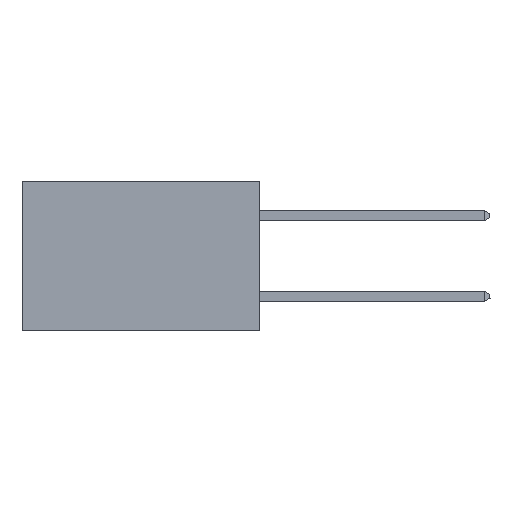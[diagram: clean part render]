
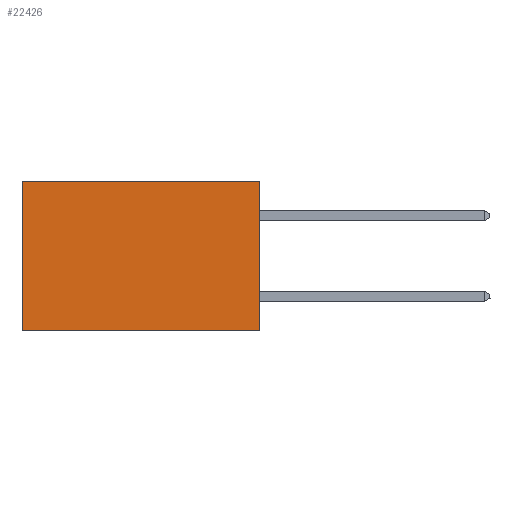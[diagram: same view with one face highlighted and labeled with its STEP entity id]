
A CAD part, left-side view. The second image highlights one B-rep face of the part: STEP entity #22426.
In plain terms, the highlighted planar face has unit normal (-1, 0, 0).
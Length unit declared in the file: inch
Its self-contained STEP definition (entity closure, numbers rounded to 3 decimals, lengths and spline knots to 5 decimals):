
#252 = DIRECTION ( 'NONE',  ( 0., 0., -1. ) ) ;
#736 = VECTOR ( 'NONE', #252, 39.37008 ) ;
#1738 = CARTESIAN_POINT ( 'NONE',  ( 0.277, 0., -0.37 ) ) ;
#1984 = CARTESIAN_POINT ( 'NONE',  ( 0.277, 0., 0. ) ) ;
#2696 = CARTESIAN_POINT ( 'NONE',  ( 0.277, 0.59, -0.37 ) ) ;
#3974 = PLANE ( 'NONE',  #16552 ) ;
#6568 = DIRECTION ( 'NONE',  ( 1., 0., 0. ) ) ;
#7200 = VECTOR ( 'NONE', #10506, 39.37008 ) ;
#7933 = CARTESIAN_POINT ( 'NONE',  ( 0.277, 0., -0.37 ) ) ;
#8193 = CARTESIAN_POINT ( 'NONE',  ( 0.277, 0.59, 0. ) ) ;
#9476 = DIRECTION ( 'NONE',  ( 0., 1., 0. ) ) ;
#10140 = VERTEX_POINT ( 'NONE', #2696 ) ;
#10506 = DIRECTION ( 'NONE',  ( 0., 0., -1. ) ) ;
#10649 = VERTEX_POINT ( 'NONE', #8193 ) ;
#10927 = EDGE_CURVE ( 'NONE', #25287, #30603, #21555, .T. ) ;
#11053 = ORIENTED_EDGE ( 'NONE', *, *, #25006, .T. ) ;
#11195 = EDGE_LOOP ( 'NONE', ( #11053, #23237, #11790, #12079 ) ) ;
#11321 = VECTOR ( 'NONE', #9476, 39.37008 ) ;
#11790 = ORIENTED_EDGE ( 'NONE', *, *, #10927, .F. ) ;
#12079 = ORIENTED_EDGE ( 'NONE', *, *, #24498, .T. ) ;
#13975 = CARTESIAN_POINT ( 'NONE',  ( 0.277, 0., 0. ) ) ;
#15087 = EDGE_CURVE ( 'NONE', #30603, #10140, #18902, .T. ) ;
#15189 = CARTESIAN_POINT ( 'NONE',  ( 0.277, 0., -0.37 ) ) ;
#16552 = AXIS2_PLACEMENT_3D ( 'NONE', #21847, #6568, #24309 ) ;
#18902 = LINE ( 'NONE', #1738, #11321 ) ;
#19803 = FACE_OUTER_BOUND ( 'NONE', #11195, .T. ) ;
#20900 = CARTESIAN_POINT ( 'NONE',  ( 0.277, 0.59, -0.37 ) ) ;
#21196 = LINE ( 'NONE', #20900, #736 ) ;
#21555 = LINE ( 'NONE', #7933, #7200 ) ;
#21847 = CARTESIAN_POINT ( 'NONE',  ( 0.277, 0., -0.37 ) ) ;
#22028 = VECTOR ( 'NONE', #28992, 39.37008 ) ;
#22426 = ADVANCED_FACE ( 'NONE', ( #19803 ), #3974, .F. ) ;
#23237 = ORIENTED_EDGE ( 'NONE', *, *, #15087, .F. ) ;
#24309 = DIRECTION ( 'NONE',  ( 0., 0., -1. ) ) ;
#24498 = EDGE_CURVE ( 'NONE', #25287, #10649, #28611, .T. ) ;
#25006 = EDGE_CURVE ( 'NONE', #10649, #10140, #21196, .T. ) ;
#25287 = VERTEX_POINT ( 'NONE', #1984 ) ;
#28611 = LINE ( 'NONE', #13975, #22028 ) ;
#28992 = DIRECTION ( 'NONE',  ( 0., 1., 0. ) ) ;
#30603 = VERTEX_POINT ( 'NONE', #15189 ) ;
